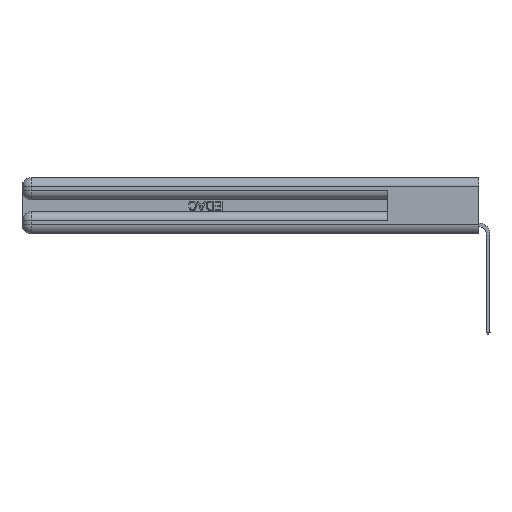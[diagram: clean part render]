
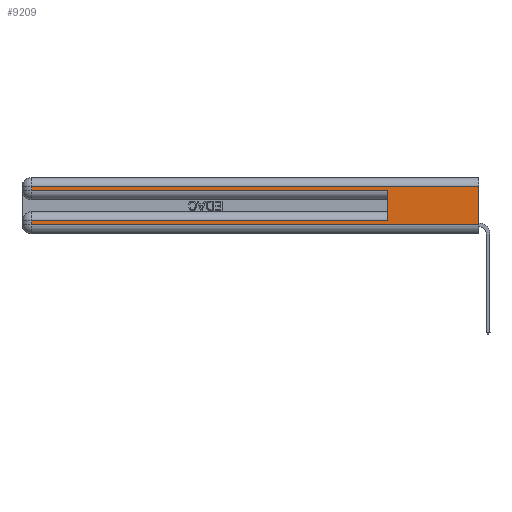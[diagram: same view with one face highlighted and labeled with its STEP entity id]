
A CAD part, left-side view. The second image highlights one B-rep face of the part: STEP entity #9209.
In plain terms, the highlighted planar face has unit normal (-1, 0, 0).
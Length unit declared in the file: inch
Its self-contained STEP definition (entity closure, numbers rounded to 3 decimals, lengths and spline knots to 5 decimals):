
#584 = DIRECTION ( 'NONE',  ( 0., 1., 0. ) ) ;
#653 = DIRECTION ( 'NONE',  ( 0., -1., 0. ) ) ;
#1526 = DIRECTION ( 'NONE',  ( 0., 1., 0. ) ) ;
#1750 = VECTOR ( 'NONE', #21708, 39.37008 ) ;
#2230 = ORIENTED_EDGE ( 'NONE', *, *, #26970, .T. ) ;
#3032 = CARTESIAN_POINT ( 'NONE',  ( 0., 0.6, 0.145 ) ) ;
#3125 = CARTESIAN_POINT ( 'NONE',  ( 0., 0., 0.06 ) ) ;
#3753 = ORIENTED_EDGE ( 'NONE', *, *, #20666, .T. ) ;
#4321 = VERTEX_POINT ( 'NONE', #11562 ) ;
#4571 = DIRECTION ( 'NONE',  ( 0., 0., -1. ) ) ;
#4866 = ORIENTED_EDGE ( 'NONE', *, *, #9490, .F. ) ;
#6126 = VERTEX_POINT ( 'NONE', #19651 ) ;
#7079 = VECTOR ( 'NONE', #653, 39.37008 ) ;
#7771 = LINE ( 'NONE', #18308, #19703 ) ;
#8038 = VECTOR ( 'NONE', #29132, 39.37008 ) ;
#8418 = VERTEX_POINT ( 'NONE', #12700 ) ;
#8796 = DIRECTION ( 'NONE',  ( 0., 0., -1. ) ) ;
#9209 = ADVANCED_FACE ( 'NONE', ( #11174 ), #10791, .F. ) ;
#9490 = EDGE_CURVE ( 'NONE', #9711, #8418, #21177, .T. ) ;
#9711 = VERTEX_POINT ( 'NONE', #9856 ) ;
#9856 = CARTESIAN_POINT ( 'NONE',  ( 0., 0., 0.31 ) ) ;
#10519 = AXIS2_PLACEMENT_3D ( 'NONE', #24772, #13203, #29721 ) ;
#10791 = PLANE ( 'NONE',  #10519 ) ;
#11111 = EDGE_CURVE ( 'NONE', #9711, #4321, #13996, .T. ) ;
#11174 = FACE_OUTER_BOUND ( 'NONE', #15640, .T. ) ;
#11301 = CARTESIAN_POINT ( 'NONE',  ( 0., 2.94, 0.37 ) ) ;
#11562 = CARTESIAN_POINT ( 'NONE',  ( 0., 2.94, 0.31 ) ) ;
#12690 = EDGE_CURVE ( 'NONE', #4321, #22365, #14282, .T. ) ;
#12700 = CARTESIAN_POINT ( 'NONE',  ( 0., 0., 0.06 ) ) ;
#12999 = CARTESIAN_POINT ( 'NONE',  ( 0., 2.94, 0.285 ) ) ;
#13203 = DIRECTION ( 'NONE',  ( 1., 0., 0. ) ) ;
#13783 = LINE ( 'NONE', #3125, #1750 ) ;
#13996 = LINE ( 'NONE', #17391, #26573 ) ;
#14246 = ORIENTED_EDGE ( 'NONE', *, *, #17486, .F. ) ;
#14282 = LINE ( 'NONE', #11301, #19115 ) ;
#14292 = EDGE_CURVE ( 'NONE', #22365, #30160, #30805, .T. ) ;
#14844 = VECTOR ( 'NONE', #4571, 39.37008 ) ;
#15046 = CARTESIAN_POINT ( 'NONE',  ( 0., 0., 0.285 ) ) ;
#15640 = EDGE_LOOP ( 'NONE', ( #4866, #23858, #30861, #19079, #14246, #26825, #2230, #3753 ) ) ;
#15879 = EDGE_CURVE ( 'NONE', #6126, #30252, #7771, .T. ) ;
#17391 = CARTESIAN_POINT ( 'NONE',  ( 0., 0., 0.31 ) ) ;
#17486 = EDGE_CURVE ( 'NONE', #6126, #30160, #19986, .T. ) ;
#18032 = CARTESIAN_POINT ( 'NONE',  ( 0., 2.94, 0.06 ) ) ;
#18301 = CARTESIAN_POINT ( 'NONE',  ( 0., 2.94, 0.37 ) ) ;
#18308 = CARTESIAN_POINT ( 'NONE',  ( 0., 0., 0.085 ) ) ;
#18897 = CARTESIAN_POINT ( 'NONE',  ( 0., 0., 0.37 ) ) ;
#19079 = ORIENTED_EDGE ( 'NONE', *, *, #14292, .T. ) ;
#19115 = VECTOR ( 'NONE', #20552, 39.37008 ) ;
#19651 = CARTESIAN_POINT ( 'NONE',  ( 0., 0.6, 0.085 ) ) ;
#19703 = VECTOR ( 'NONE', #1526, 39.37008 ) ;
#19986 = LINE ( 'NONE', #3032, #8038 ) ;
#20253 = VERTEX_POINT ( 'NONE', #18032 ) ;
#20552 = DIRECTION ( 'NONE',  ( 0., 0., -1. ) ) ;
#20666 = EDGE_CURVE ( 'NONE', #20253, #8418, #13783, .T. ) ;
#21177 = LINE ( 'NONE', #18897, #14844 ) ;
#21708 = DIRECTION ( 'NONE',  ( 0., -1., 0. ) ) ;
#22365 = VERTEX_POINT ( 'NONE', #12999 ) ;
#22974 = VECTOR ( 'NONE', #8796, 39.37008 ) ;
#23858 = ORIENTED_EDGE ( 'NONE', *, *, #11111, .T. ) ;
#24772 = CARTESIAN_POINT ( 'NONE',  ( 0., 0., 0.37 ) ) ;
#26573 = VECTOR ( 'NONE', #584, 39.37008 ) ;
#26825 = ORIENTED_EDGE ( 'NONE', *, *, #15879, .T. ) ;
#26970 = EDGE_CURVE ( 'NONE', #30252, #20253, #29244, .T. ) ;
#29132 = DIRECTION ( 'NONE',  ( 0., 0., 1. ) ) ;
#29244 = LINE ( 'NONE', #18301, #22974 ) ;
#29721 = DIRECTION ( 'NONE',  ( 0., 0., -1. ) ) ;
#29815 = CARTESIAN_POINT ( 'NONE',  ( 0., 0.6, 0.285 ) ) ;
#30160 = VERTEX_POINT ( 'NONE', #29815 ) ;
#30252 = VERTEX_POINT ( 'NONE', #30727 ) ;
#30727 = CARTESIAN_POINT ( 'NONE',  ( 0., 2.94, 0.085 ) ) ;
#30805 = LINE ( 'NONE', #15046, #7079 ) ;
#30861 = ORIENTED_EDGE ( 'NONE', *, *, #12690, .T. ) ;
